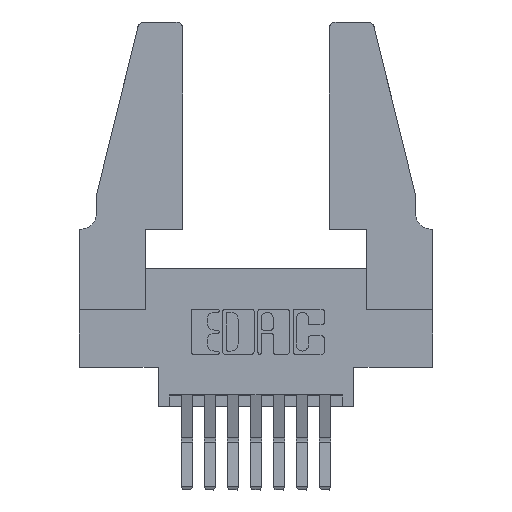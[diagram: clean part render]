
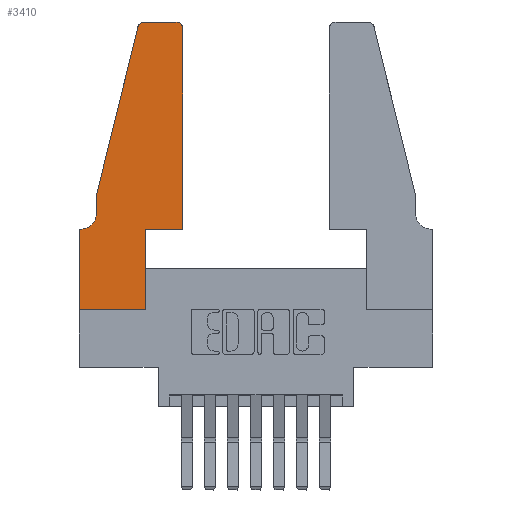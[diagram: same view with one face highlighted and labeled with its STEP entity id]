
A CAD part, top view. The second image highlights one B-rep face of the part: STEP entity #3410.
In plain terms, the highlighted planar face has unit normal (0, 0, 1).
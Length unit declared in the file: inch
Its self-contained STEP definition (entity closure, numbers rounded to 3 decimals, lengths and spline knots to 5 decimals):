
#4 = ORIENTED_EDGE ( 'NONE', *, *, #3317, .T. ) ;
#9 = VERTEX_POINT ( 'NONE', #375 ) ;
#68 = EDGE_CURVE ( 'NONE', #3512, #2507, #10279, .T. ) ;
#375 = CARTESIAN_POINT ( 'NONE',  ( 0., 0.35, 0.37 ) ) ;
#488 = CARTESIAN_POINT ( 'NONE',  ( 0.0055, 0.42, 0.37 ) ) ;
#735 = LINE ( 'NONE', #8961, #10831 ) ;
#842 = CARTESIAN_POINT ( 'NONE',  ( 0.0055, 0.35, 0.37 ) ) ;
#979 = LINE ( 'NONE', #2127, #11023 ) ;
#1024 = CIRCLE ( 'NONE', #8184, 0.03 ) ;
#1046 = VERTEX_POINT ( 'NONE', #8003 ) ;
#1065 = DIRECTION ( 'NONE',  ( -0.239, -0.971, 0. ) ) ;
#1660 = DIRECTION ( 'NONE',  ( -1., 0., 0. ) ) ;
#1780 = CARTESIAN_POINT ( 'NONE',  ( 0.284, 1.25, 0.37 ) ) ;
#1851 = CARTESIAN_POINT ( 'NONE',  ( 0.0755, 0.5, 0.37 ) ) ;
#2076 = DIRECTION ( 'NONE',  ( 0., -1., 0. ) ) ;
#2084 = VERTEX_POINT ( 'NONE', #8331 ) ;
#2127 = CARTESIAN_POINT ( 'NONE',  ( 0.2865, 0.35, 0.37 ) ) ;
#2306 = ORIENTED_EDGE ( 'NONE', *, *, #11403, .T. ) ;
#2382 = CARTESIAN_POINT ( 'NONE',  ( 0., 0., 0.37 ) ) ;
#2507 = VERTEX_POINT ( 'NONE', #1780 ) ;
#2535 = DIRECTION ( 'NONE',  ( 0., 0., 1. ) ) ;
#2695 = DIRECTION ( 'NONE',  ( 1., 0., 0. ) ) ;
#2707 = CARTESIAN_POINT ( 'NONE',  ( 0.4505, 0.35, 0.37 ) ) ;
#2970 = CARTESIAN_POINT ( 'NONE',  ( 0.4205, 1.25, 0.37 ) ) ;
#3006 = CARTESIAN_POINT ( 'NONE',  ( 0.0755, 0.35, 0.37 ) ) ;
#3229 = VECTOR ( 'NONE', #3754, 39.37008 ) ;
#3317 = EDGE_CURVE ( 'NONE', #9, #4658, #6245, .T. ) ;
#3410 = ADVANCED_FACE ( 'NONE', ( #12391 ), #4265, .T. ) ;
#3439 = ORIENTED_EDGE ( 'NONE', *, *, #10046, .T. ) ;
#3512 = VERTEX_POINT ( 'NONE', #2970 ) ;
#3635 = EDGE_CURVE ( 'NONE', #5571, #8156, #8006, .T. ) ;
#3754 = DIRECTION ( 'NONE',  ( 1., 0., 0. ) ) ;
#3931 = VECTOR ( 'NONE', #2695, 39.37008 ) ;
#4018 = CARTESIAN_POINT ( 'NONE',  ( 0.25487, 1.22718, 0.37 ) ) ;
#4098 = LINE ( 'NONE', #6840, #6284 ) ;
#4170 = DIRECTION ( 'NONE',  ( 1., 0., 0. ) ) ;
#4186 = DIRECTION ( 'NONE',  ( 0., 0., 1. ) ) ;
#4194 = CARTESIAN_POINT ( 'NONE',  ( 0., 0.35, 0.37 ) ) ;
#4265 = PLANE ( 'NONE',  #11561 ) ;
#4371 = VERTEX_POINT ( 'NONE', #842 ) ;
#4396 = VECTOR ( 'NONE', #8738, 39.37008 ) ;
#4658 = VERTEX_POINT ( 'NONE', #2382 ) ;
#4905 = ORIENTED_EDGE ( 'NONE', *, *, #7446, .T. ) ;
#5008 = AXIS2_PLACEMENT_3D ( 'NONE', #488, #7576, #1660 ) ;
#5142 = EDGE_CURVE ( 'NONE', #11565, #5571, #735, .T. ) ;
#5176 = CARTESIAN_POINT ( 'NONE',  ( 0.2865, 0.35, 0.37 ) ) ;
#5198 = DIRECTION ( 'NONE',  ( 0., -1., 0. ) ) ;
#5223 = CARTESIAN_POINT ( 'NONE',  ( 0., 0., 0.37 ) ) ;
#5532 = ORIENTED_EDGE ( 'NONE', *, *, #3635, .T. ) ;
#5571 = VERTEX_POINT ( 'NONE', #11371 ) ;
#6072 = DIRECTION ( 'NONE',  ( 0., 0., 1. ) ) ;
#6220 = AXIS2_PLACEMENT_3D ( 'NONE', #8326, #2535, #9248 ) ;
#6245 = LINE ( 'NONE', #5223, #10871 ) ;
#6284 = VECTOR ( 'NONE', #9642, 39.37008 ) ;
#6427 = LINE ( 'NONE', #9372, #3931 ) ;
#6792 = CIRCLE ( 'NONE', #5008, 0.07 ) ;
#6840 = CARTESIAN_POINT ( 'NONE',  ( 0.4505, 0.35, 0.37 ) ) ;
#7035 = DIRECTION ( 'NONE',  ( 0., 1., 0. ) ) ;
#7187 = ORIENTED_EDGE ( 'NONE', *, *, #9209, .T. ) ;
#7405 = ORIENTED_EDGE ( 'NONE', *, *, #68, .T. ) ;
#7446 = EDGE_CURVE ( 'NONE', #10008, #2084, #4098, .T. ) ;
#7576 = DIRECTION ( 'NONE',  ( 0., 0., -1. ) ) ;
#7940 = CARTESIAN_POINT ( 'NONE',  ( 0.4505, 0.35, 0.37 ) ) ;
#7988 = LINE ( 'NONE', #2707, #3229 ) ;
#8003 = CARTESIAN_POINT ( 'NONE',  ( 0.2865, 0., 0.37 ) ) ;
#8006 = LINE ( 'NONE', #1851, #10170 ) ;
#8100 = EDGE_CURVE ( 'NONE', #4371, #9, #11458, .T. ) ;
#8156 = VERTEX_POINT ( 'NONE', #9707 ) ;
#8184 = AXIS2_PLACEMENT_3D ( 'NONE', #11570, #6072, #12459 ) ;
#8326 = CARTESIAN_POINT ( 'NONE',  ( 0.284, 1.22, 0.37 ) ) ;
#8331 = CARTESIAN_POINT ( 'NONE',  ( 0.4505, 1.22, 0.37 ) ) ;
#8738 = DIRECTION ( 'NONE',  ( -1., 0., 0. ) ) ;
#8869 = EDGE_CURVE ( 'NONE', #2084, #3512, #1024, .T. ) ;
#8961 = CARTESIAN_POINT ( 'NONE',  ( 0.0755, 0.5, 0.37 ) ) ;
#9209 = EDGE_CURVE ( 'NONE', #4658, #1046, #6427, .T. ) ;
#9248 = DIRECTION ( 'NONE',  ( 1., 0., 0. ) ) ;
#9372 = CARTESIAN_POINT ( 'NONE',  ( 0., 0., 0.37 ) ) ;
#9598 = EDGE_CURVE ( 'NONE', #2507, #11565, #11852, .T. ) ;
#9642 = DIRECTION ( 'NONE',  ( 0., 1., 0. ) ) ;
#9707 = CARTESIAN_POINT ( 'NONE',  ( 0.0755, 0.42, 0.37 ) ) ;
#9877 = DIRECTION ( 'NONE',  ( -1., 0., 0. ) ) ;
#9988 = VECTOR ( 'NONE', #9877, 39.37008 ) ;
#10008 = VERTEX_POINT ( 'NONE', #7940 ) ;
#10046 = EDGE_CURVE ( 'NONE', #1046, #10487, #979, .T. ) ;
#10085 = ORIENTED_EDGE ( 'NONE', *, *, #9598, .T. ) ;
#10170 = VECTOR ( 'NONE', #2076, 39.37008 ) ;
#10279 = LINE ( 'NONE', #11318, #9988 ) ;
#10487 = VERTEX_POINT ( 'NONE', #5176 ) ;
#10588 = EDGE_LOOP ( 'NONE', ( #7405, #10085, #11810, #5532, #11047, #12120, #4, #7187, #3439, #2306, #4905, #12426 ) ) ;
#10831 = VECTOR ( 'NONE', #1065, 39.37008 ) ;
#10871 = VECTOR ( 'NONE', #5198, 39.37008 ) ;
#11023 = VECTOR ( 'NONE', #7035, 39.37008 ) ;
#11047 = ORIENTED_EDGE ( 'NONE', *, *, #11918, .T. ) ;
#11318 = CARTESIAN_POINT ( 'NONE',  ( 0.2605, 1.25, 0.37 ) ) ;
#11371 = CARTESIAN_POINT ( 'NONE',  ( 0.0755, 0.5, 0.37 ) ) ;
#11403 = EDGE_CURVE ( 'NONE', #10487, #10008, #7988, .T. ) ;
#11458 = LINE ( 'NONE', #3006, #4396 ) ;
#11561 = AXIS2_PLACEMENT_3D ( 'NONE', #4194, #4186, #4170 ) ;
#11565 = VERTEX_POINT ( 'NONE', #4018 ) ;
#11570 = CARTESIAN_POINT ( 'NONE',  ( 0.4205, 1.22, 0.37 ) ) ;
#11810 = ORIENTED_EDGE ( 'NONE', *, *, #5142, .T. ) ;
#11852 = CIRCLE ( 'NONE', #6220, 0.03 ) ;
#11918 = EDGE_CURVE ( 'NONE', #8156, #4371, #6792, .T. ) ;
#12120 = ORIENTED_EDGE ( 'NONE', *, *, #8100, .T. ) ;
#12391 = FACE_OUTER_BOUND ( 'NONE', #10588, .T. ) ;
#12426 = ORIENTED_EDGE ( 'NONE', *, *, #8869, .T. ) ;
#12459 = DIRECTION ( 'NONE',  ( 1., 0., 0. ) ) ;
